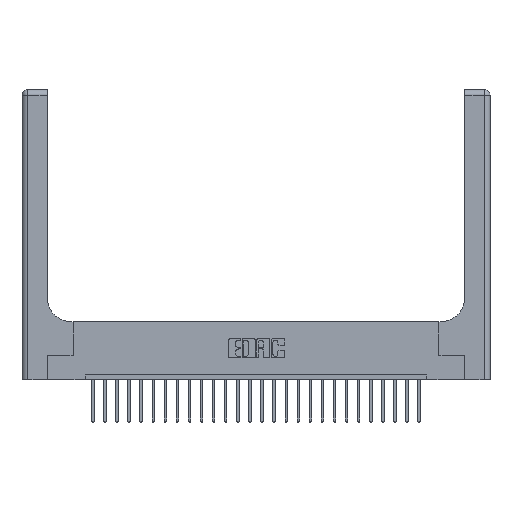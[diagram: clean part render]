
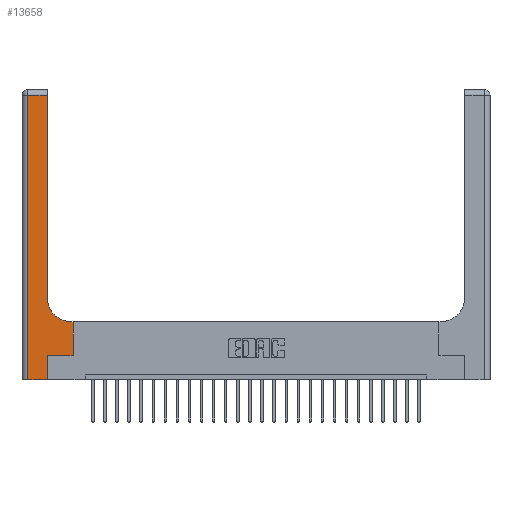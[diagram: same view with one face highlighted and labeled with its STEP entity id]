
A CAD part, top view. The second image highlights one B-rep face of the part: STEP entity #13658.
In plain terms, the highlighted planar face has unit normal (0, 0, 1).
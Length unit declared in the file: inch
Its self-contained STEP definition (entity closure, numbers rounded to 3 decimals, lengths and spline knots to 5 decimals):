
#425 = VERTEX_POINT ( 'NONE', #11912 ) ;
#464 = DIRECTION ( 'NONE',  ( 0., 1., 0. ) ) ;
#514 = EDGE_CURVE ( 'NONE', #425, #9922, #19761, .T. ) ;
#1465 = FACE_OUTER_BOUND ( 'NONE', #3822, .T. ) ;
#1573 = EDGE_CURVE ( 'NONE', #8903, #7764, #15931, .T. ) ;
#2534 = DIRECTION ( 'NONE',  ( 1., 0., 0. ) ) ;
#2638 = AXIS2_PLACEMENT_3D ( 'NONE', #8906, #9158, #14553 ) ;
#3018 = EDGE_CURVE ( 'NONE', #7764, #19990, #3026, .T. ) ;
#3026 = LINE ( 'NONE', #5033, #14741 ) ;
#3822 = EDGE_LOOP ( 'NONE', ( #13340, #16067, #14249, #13775, #5665, #12290, #18752, #10019, #22496 ) ) ;
#4025 = VECTOR ( 'NONE', #464, 39.37008 ) ;
#4077 = VERTEX_POINT ( 'NONE', #8218 ) ;
#4532 = LINE ( 'NONE', #23578, #19393 ) ;
#4871 = DIRECTION ( 'NONE',  ( 0., 1., 0. ) ) ;
#5033 = CARTESIAN_POINT ( 'NONE',  ( 0., 0., 0.37 ) ) ;
#5665 = ORIENTED_EDGE ( 'NONE', *, *, #19001, .T. ) ;
#5683 = DIRECTION ( 'NONE',  ( -1., 0., 0. ) ) ;
#6196 = EDGE_CURVE ( 'NONE', #15692, #4077, #4532, .T. ) ;
#6254 = CARTESIAN_POINT ( 'NONE',  ( 0.06, 3., 0.37 ) ) ;
#6298 = VECTOR ( 'NONE', #5683, 39.37008 ) ;
#7111 = EDGE_CURVE ( 'NONE', #4077, #15205, #12999, .T. ) ;
#7336 = EDGE_CURVE ( 'NONE', #9011, #8903, #17029, .T. ) ;
#7626 = VECTOR ( 'NONE', #4871, 39.37008 ) ;
#7764 = VERTEX_POINT ( 'NONE', #17725 ) ;
#8218 = CARTESIAN_POINT ( 'NONE',  ( 0.528, 0.25, 0.37 ) ) ;
#8341 = CARTESIAN_POINT ( 'NONE',  ( 0.265, 0., 0.37 ) ) ;
#8903 = VERTEX_POINT ( 'NONE', #23684 ) ;
#8906 = CARTESIAN_POINT ( 'NONE',  ( 0., 3., 0.37 ) ) ;
#9011 = VERTEX_POINT ( 'NONE', #14218 ) ;
#9158 = DIRECTION ( 'NONE',  ( 0., 0., -1. ) ) ;
#9771 = CARTESIAN_POINT ( 'NONE',  ( 0.528, 0.6, 0.37 ) ) ;
#9922 = VERTEX_POINT ( 'NONE', #13736 ) ;
#10019 = ORIENTED_EDGE ( 'NONE', *, *, #23953, .T. ) ;
#10682 = VECTOR ( 'NONE', #13935, 39.37008 ) ;
#10704 = DIRECTION ( 'NONE',  ( 1., 0., 0. ) ) ;
#11912 = CARTESIAN_POINT ( 'NONE',  ( 0.51, 0.6, 0.37 ) ) ;
#12290 = ORIENTED_EDGE ( 'NONE', *, *, #6196, .T. ) ;
#12999 = LINE ( 'NONE', #18284, #21136 ) ;
#13340 = ORIENTED_EDGE ( 'NONE', *, *, #19240, .T. ) ;
#13658 = ADVANCED_FACE ( 'NONE', ( #1465 ), #24144, .F. ) ;
#13736 = CARTESIAN_POINT ( 'NONE',  ( 0.26, 0.85, 0.37 ) ) ;
#13775 = ORIENTED_EDGE ( 'NONE', *, *, #3018, .T. ) ;
#13916 = CARTESIAN_POINT ( 'NONE',  ( 0.26, 3., 0.37 ) ) ;
#13935 = DIRECTION ( 'NONE',  ( 0., -1., 0. ) ) ;
#14218 = CARTESIAN_POINT ( 'NONE',  ( 0.26, 2.94, 0.37 ) ) ;
#14249 = ORIENTED_EDGE ( 'NONE', *, *, #1573, .T. ) ;
#14472 = CARTESIAN_POINT ( 'NONE',  ( 0.265, 0.25, 0.37 ) ) ;
#14553 = DIRECTION ( 'NONE',  ( -1., 0., 0. ) ) ;
#14741 = VECTOR ( 'NONE', #10704, 39.37008 ) ;
#14816 = CARTESIAN_POINT ( 'NONE',  ( 0.26, 0.6, 0.37 ) ) ;
#15055 = DIRECTION ( 'NONE',  ( -1., 0., 0. ) ) ;
#15205 = VERTEX_POINT ( 'NONE', #9771 ) ;
#15692 = VERTEX_POINT ( 'NONE', #14472 ) ;
#15852 = CARTESIAN_POINT ( 'NONE',  ( 0.265, 0., 0.37 ) ) ;
#15931 = LINE ( 'NONE', #6254, #10682 ) ;
#16067 = ORIENTED_EDGE ( 'NONE', *, *, #7336, .T. ) ;
#16951 = LINE ( 'NONE', #14816, #24677 ) ;
#17029 = LINE ( 'NONE', #17257, #6298 ) ;
#17257 = CARTESIAN_POINT ( 'NONE',  ( 0., 2.94, 0.37 ) ) ;
#17683 = LINE ( 'NONE', #13916, #4025 ) ;
#17725 = CARTESIAN_POINT ( 'NONE',  ( 0.06, 0., 0.37 ) ) ;
#18284 = CARTESIAN_POINT ( 'NONE',  ( 0.528, 0.25, 0.37 ) ) ;
#18700 = DIRECTION ( 'NONE',  ( 0., 0., -1. ) ) ;
#18752 = ORIENTED_EDGE ( 'NONE', *, *, #7111, .T. ) ;
#19001 = EDGE_CURVE ( 'NONE', #19990, #15692, #24162, .T. ) ;
#19240 = EDGE_CURVE ( 'NONE', #9922, #9011, #17683, .T. ) ;
#19393 = VECTOR ( 'NONE', #2534, 39.37008 ) ;
#19761 = CIRCLE ( 'NONE', #20574, 0.25 ) ;
#19990 = VERTEX_POINT ( 'NONE', #8341 ) ;
#20574 = AXIS2_PLACEMENT_3D ( 'NONE', #24525, #18700, #24271 ) ;
#21136 = VECTOR ( 'NONE', #22710, 39.37008 ) ;
#22496 = ORIENTED_EDGE ( 'NONE', *, *, #514, .T. ) ;
#22710 = DIRECTION ( 'NONE',  ( 0., 1., 0. ) ) ;
#23578 = CARTESIAN_POINT ( 'NONE',  ( 0.265, 0.25, 0.37 ) ) ;
#23684 = CARTESIAN_POINT ( 'NONE',  ( 0.06, 2.94, 0.37 ) ) ;
#23953 = EDGE_CURVE ( 'NONE', #15205, #425, #16951, .T. ) ;
#24144 = PLANE ( 'NONE',  #2638 ) ;
#24162 = LINE ( 'NONE', #15852, #7626 ) ;
#24271 = DIRECTION ( 'NONE',  ( 1., 0., 0. ) ) ;
#24525 = CARTESIAN_POINT ( 'NONE',  ( 0.51, 0.85, 0.37 ) ) ;
#24677 = VECTOR ( 'NONE', #15055, 39.37008 ) ;
